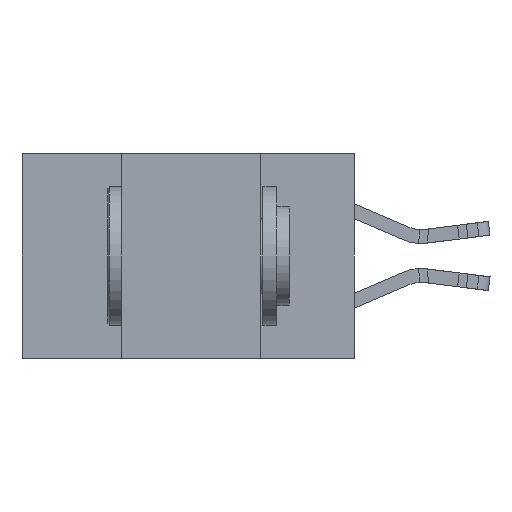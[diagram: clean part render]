
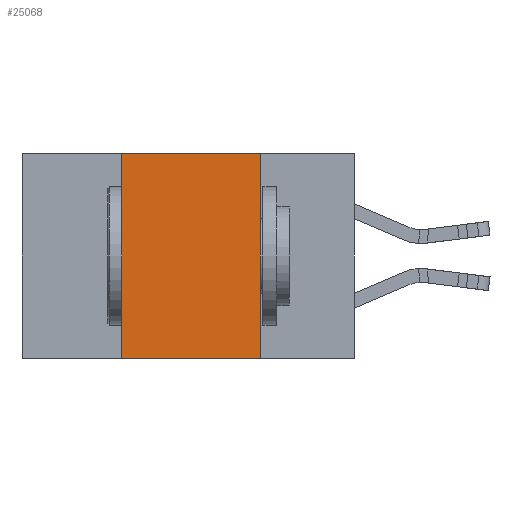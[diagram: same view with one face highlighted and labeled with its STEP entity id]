
A CAD part, left-side view. The second image highlights one B-rep face of the part: STEP entity #25068.
In plain terms, the highlighted planar face has unit normal (-1, 0, 0).
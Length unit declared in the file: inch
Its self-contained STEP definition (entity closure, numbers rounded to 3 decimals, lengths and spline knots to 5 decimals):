
#339 = CARTESIAN_POINT ( 'NONE',  ( 0., 0.6, 0. ) ) ;
#1918 = VECTOR ( 'NONE', #3976, 39.37008 ) ;
#3003 = ORIENTED_EDGE ( 'NONE', *, *, #20339, .F. ) ;
#3976 = DIRECTION ( 'NONE',  ( 0., -1., 0. ) ) ;
#5330 = LINE ( 'NONE', #23685, #21936 ) ;
#7277 = AXIS2_PLACEMENT_3D ( 'NONE', #339, #20705, #11715 ) ;
#7484 = CARTESIAN_POINT ( 'NONE',  ( 0., 0.17, -0.37 ) ) ;
#9385 = PLANE ( 'NONE',  #7277 ) ;
#10796 = CARTESIAN_POINT ( 'NONE',  ( 0., 0.17, 0. ) ) ;
#11279 = EDGE_CURVE ( 'NONE', #20492, #27503, #21743, .T. ) ;
#11715 = DIRECTION ( 'NONE',  ( 0., 0., -1. ) ) ;
#12102 = CARTESIAN_POINT ( 'NONE',  ( 0., 0.42, -0.37 ) ) ;
#12190 = DIRECTION ( 'NONE',  ( 0., 0., 1. ) ) ;
#12528 = ORIENTED_EDGE ( 'NONE', *, *, #25747, .F. ) ;
#13645 = FACE_OUTER_BOUND ( 'NONE', #17507, .T. ) ;
#15041 = LINE ( 'NONE', #29496, #24809 ) ;
#15238 = ORIENTED_EDGE ( 'NONE', *, *, #11279, .T. ) ;
#15687 = DIRECTION ( 'NONE',  ( 0., -1., 0. ) ) ;
#17393 = ORIENTED_EDGE ( 'NONE', *, *, #25963, .F. ) ;
#17507 = EDGE_LOOP ( 'NONE', ( #3003, #17393, #12528, #15238 ) ) ;
#18407 = VERTEX_POINT ( 'NONE', #25335 ) ;
#20339 = EDGE_CURVE ( 'NONE', #18407, #27503, #26103, .T. ) ;
#20492 = VERTEX_POINT ( 'NONE', #12102 ) ;
#20705 = DIRECTION ( 'NONE',  ( 1., 0., 0. ) ) ;
#21067 = VECTOR ( 'NONE', #29247, 39.37008 ) ;
#21743 = LINE ( 'NONE', #29238, #1918 ) ;
#21936 = VECTOR ( 'NONE', #12190, 39.37008 ) ;
#21998 = CARTESIAN_POINT ( 'NONE',  ( 0., 0.42, 0. ) ) ;
#23685 = CARTESIAN_POINT ( 'NONE',  ( 0., 0.42, 0. ) ) ;
#24809 = VECTOR ( 'NONE', #15687, 39.37008 ) ;
#25068 = ADVANCED_FACE ( 'NONE', ( #13645 ), #9385, .F. ) ;
#25335 = CARTESIAN_POINT ( 'NONE',  ( 0., 0.17, 0. ) ) ;
#25747 = EDGE_CURVE ( 'NONE', #20492, #27951, #5330, .T. ) ;
#25963 = EDGE_CURVE ( 'NONE', #27951, #18407, #15041, .T. ) ;
#26103 = LINE ( 'NONE', #10796, #21067 ) ;
#27503 = VERTEX_POINT ( 'NONE', #7484 ) ;
#27951 = VERTEX_POINT ( 'NONE', #21998 ) ;
#29238 = CARTESIAN_POINT ( 'NONE',  ( 0., 0.6, -0.37 ) ) ;
#29247 = DIRECTION ( 'NONE',  ( 0., 0., -1. ) ) ;
#29496 = CARTESIAN_POINT ( 'NONE',  ( 0., 0.6, 0. ) ) ;
